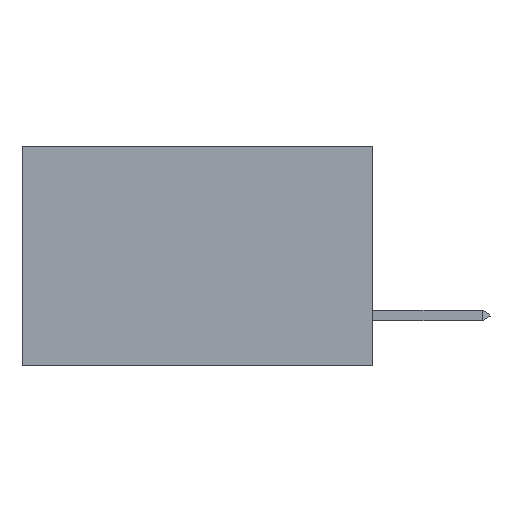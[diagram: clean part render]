
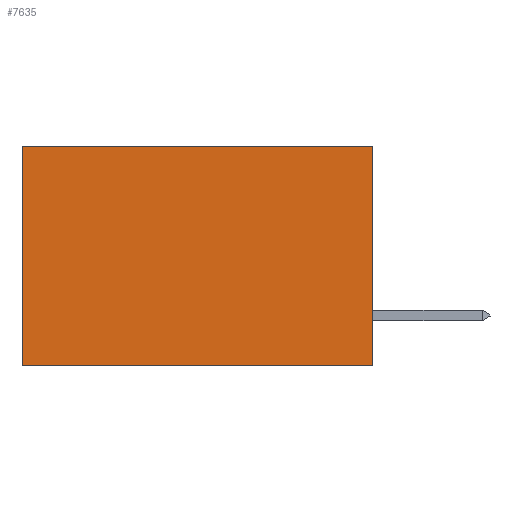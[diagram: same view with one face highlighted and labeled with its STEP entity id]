
A CAD part, left-side view. The second image highlights one B-rep face of the part: STEP entity #7635.
In plain terms, the highlighted planar face has unit normal (-1, 0, 0).
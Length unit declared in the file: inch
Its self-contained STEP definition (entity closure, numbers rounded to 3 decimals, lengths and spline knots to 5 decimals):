
#85 = VECTOR ( 'NONE', #16437, 39.37008 ) ;
#253 = DIRECTION ( 'NONE',  ( 0., 1., 0. ) ) ;
#492 = CARTESIAN_POINT ( 'NONE',  ( 0.277, 0., -0.37 ) ) ;
#511 = DIRECTION ( 'NONE',  ( 0., 0., -1. ) ) ;
#517 = AXIS2_PLACEMENT_3D ( 'NONE', #15848, #10055, #511 ) ;
#1867 = LINE ( 'NONE', #19329, #13694 ) ;
#2011 = LINE ( 'NONE', #12936, #5834 ) ;
#2119 = ORIENTED_EDGE ( 'NONE', *, *, #5931, .F. ) ;
#3058 = VERTEX_POINT ( 'NONE', #12151 ) ;
#3069 = CARTESIAN_POINT ( 'NONE',  ( 0.277, 0., 0. ) ) ;
#3887 = LINE ( 'NONE', #5955, #85 ) ;
#5338 = DIRECTION ( 'NONE',  ( 0., 1., 0. ) ) ;
#5356 = PLANE ( 'NONE',  #517 ) ;
#5834 = VECTOR ( 'NONE', #5338, 39.37008 ) ;
#5931 = EDGE_CURVE ( 'NONE', #8425, #17902, #14240, .T. ) ;
#5955 = CARTESIAN_POINT ( 'NONE',  ( 0.277, 0.59, -0.37 ) ) ;
#6090 = CARTESIAN_POINT ( 'NONE',  ( 0.277, 0., -0.37 ) ) ;
#6297 = VECTOR ( 'NONE', #253, 39.37008 ) ;
#6945 = ORIENTED_EDGE ( 'NONE', *, *, #10605, .T. ) ;
#7635 = ADVANCED_FACE ( 'NONE', ( #11896 ), #5356, .F. ) ;
#8376 = EDGE_CURVE ( 'NONE', #3058, #17902, #3887, .T. ) ;
#8425 = VERTEX_POINT ( 'NONE', #6090 ) ;
#8623 = ORIENTED_EDGE ( 'NONE', *, *, #8376, .T. ) ;
#9408 = VERTEX_POINT ( 'NONE', #3069 ) ;
#10055 = DIRECTION ( 'NONE',  ( 1., 0., 0. ) ) ;
#10605 = EDGE_CURVE ( 'NONE', #9408, #3058, #2011, .T. ) ;
#10701 = DIRECTION ( 'NONE',  ( 0., 0., -1. ) ) ;
#11896 = FACE_OUTER_BOUND ( 'NONE', #17944, .T. ) ;
#12151 = CARTESIAN_POINT ( 'NONE',  ( 0.277, 0.59, 0. ) ) ;
#12936 = CARTESIAN_POINT ( 'NONE',  ( 0.277, 0., 0. ) ) ;
#13694 = VECTOR ( 'NONE', #10701, 39.37008 ) ;
#14240 = LINE ( 'NONE', #492, #6297 ) ;
#14377 = ORIENTED_EDGE ( 'NONE', *, *, #17228, .F. ) ;
#15045 = CARTESIAN_POINT ( 'NONE',  ( 0.277, 0.59, -0.37 ) ) ;
#15848 = CARTESIAN_POINT ( 'NONE',  ( 0.277, 0., -0.37 ) ) ;
#16437 = DIRECTION ( 'NONE',  ( 0., 0., -1. ) ) ;
#17228 = EDGE_CURVE ( 'NONE', #9408, #8425, #1867, .T. ) ;
#17902 = VERTEX_POINT ( 'NONE', #15045 ) ;
#17944 = EDGE_LOOP ( 'NONE', ( #8623, #2119, #14377, #6945 ) ) ;
#19329 = CARTESIAN_POINT ( 'NONE',  ( 0.277, 0., -0.37 ) ) ;
